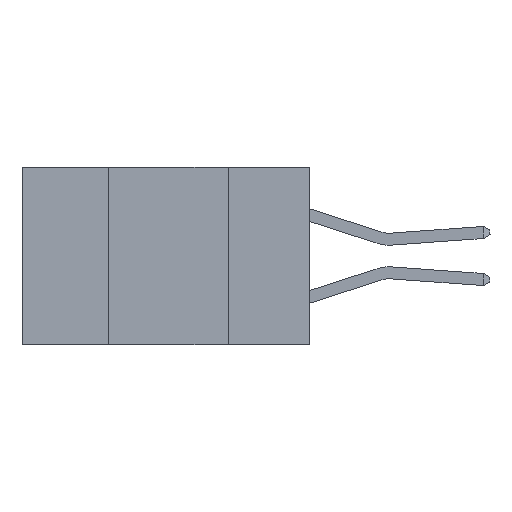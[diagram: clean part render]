
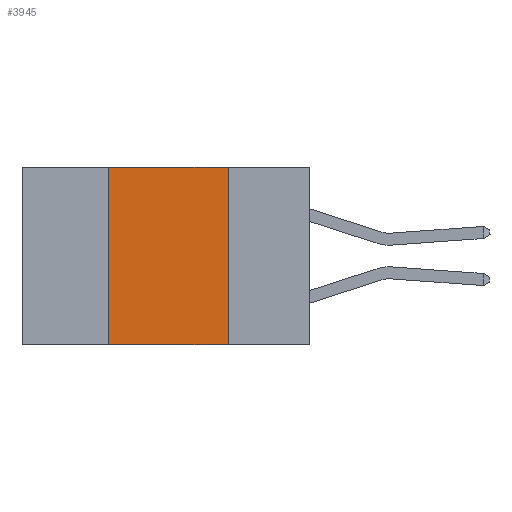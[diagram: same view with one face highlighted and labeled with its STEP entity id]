
A CAD part, left-side view. The second image highlights one B-rep face of the part: STEP entity #3945.
In plain terms, the highlighted planar face has unit normal (-1, 0, 0).
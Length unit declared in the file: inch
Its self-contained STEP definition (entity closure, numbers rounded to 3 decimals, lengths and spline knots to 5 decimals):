
#317 = ORIENTED_EDGE ( 'NONE', *, *, #9046, .F. ) ;
#634 = LINE ( 'NONE', #7397, #7413 ) ;
#694 = AXIS2_PLACEMENT_3D ( 'NONE', #6235, #9748, #957 ) ;
#957 = DIRECTION ( 'NONE',  ( 0., 0., -1. ) ) ;
#1424 = CARTESIAN_POINT ( 'NONE',  ( 0., 0.42, 0. ) ) ;
#1690 = ORIENTED_EDGE ( 'NONE', *, *, #3069, .F. ) ;
#1818 = VERTEX_POINT ( 'NONE', #1424 ) ;
#2088 = DIRECTION ( 'NONE',  ( 0., -1., 0. ) ) ;
#2931 = CARTESIAN_POINT ( 'NONE',  ( 0., 0.42, -0.37 ) ) ;
#3069 = EDGE_CURVE ( 'NONE', #1818, #5271, #634, .T. ) ;
#3379 = EDGE_CURVE ( 'NONE', #7200, #7808, #3814, .T. ) ;
#3814 = LINE ( 'NONE', #7356, #4376 ) ;
#3945 = ADVANCED_FACE ( 'NONE', ( #9747 ), #8044, .F. ) ;
#4035 = EDGE_LOOP ( 'NONE', ( #10823, #1690, #317, #4722 ) ) ;
#4361 = CARTESIAN_POINT ( 'NONE',  ( 0., 0.17, -0.37 ) ) ;
#4376 = VECTOR ( 'NONE', #10770, 39.37008 ) ;
#4662 = DIRECTION ( 'NONE',  ( 0., 0., -1. ) ) ;
#4722 = ORIENTED_EDGE ( 'NONE', *, *, #3379, .T. ) ;
#5155 = DIRECTION ( 'NONE',  ( 0., 0., 1. ) ) ;
#5271 = VERTEX_POINT ( 'NONE', #8202 ) ;
#5965 = EDGE_CURVE ( 'NONE', #5271, #7808, #7732, .T. ) ;
#6138 = VECTOR ( 'NONE', #5155, 39.37008 ) ;
#6235 = CARTESIAN_POINT ( 'NONE',  ( 0., 0.6, 0. ) ) ;
#7200 = VERTEX_POINT ( 'NONE', #2931 ) ;
#7356 = CARTESIAN_POINT ( 'NONE',  ( 0., 0.6, -0.37 ) ) ;
#7397 = CARTESIAN_POINT ( 'NONE',  ( 0., 0.6, 0. ) ) ;
#7413 = VECTOR ( 'NONE', #2088, 39.37008 ) ;
#7732 = LINE ( 'NONE', #8163, #10394 ) ;
#7751 = CARTESIAN_POINT ( 'NONE',  ( 0., 0.42, 0. ) ) ;
#7808 = VERTEX_POINT ( 'NONE', #4361 ) ;
#8044 = PLANE ( 'NONE',  #694 ) ;
#8163 = CARTESIAN_POINT ( 'NONE',  ( 0., 0.17, 0. ) ) ;
#8202 = CARTESIAN_POINT ( 'NONE',  ( 0., 0.17, 0. ) ) ;
#8790 = LINE ( 'NONE', #7751, #6138 ) ;
#9046 = EDGE_CURVE ( 'NONE', #7200, #1818, #8790, .T. ) ;
#9747 = FACE_OUTER_BOUND ( 'NONE', #4035, .T. ) ;
#9748 = DIRECTION ( 'NONE',  ( 1., 0., 0. ) ) ;
#10394 = VECTOR ( 'NONE', #4662, 39.37008 ) ;
#10770 = DIRECTION ( 'NONE',  ( 0., -1., 0. ) ) ;
#10823 = ORIENTED_EDGE ( 'NONE', *, *, #5965, .F. ) ;
